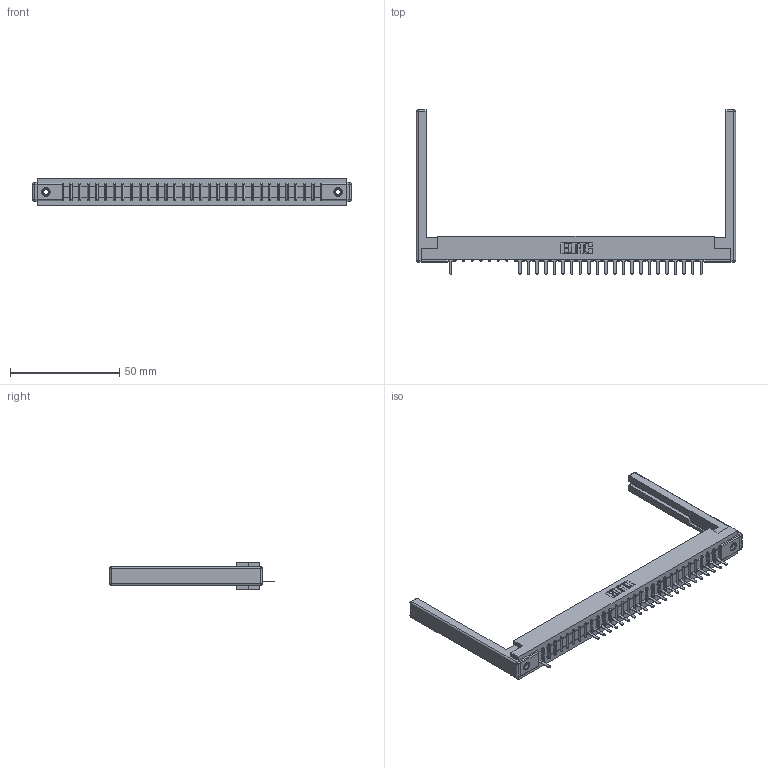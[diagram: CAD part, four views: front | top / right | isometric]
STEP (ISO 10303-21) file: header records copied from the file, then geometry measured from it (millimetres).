
FILE_DESCRIPTION (( 'STEP AP203' ), '1' );
FILE_NAME ('307-030-525-168.STEP', '2018-08-04T18:25:08', ( '' ), ( '' ), 'SwSTEP 2.0', 'SolidWorks 2016', '' );
FILE_SCHEMA (( 'CONFIG_CONTROL_DESIGN' ));
Length unit declared in the file: inch
Products named in the file (5): 307 Part_.156 Dia Mounting Holes; 307-290-001_525; 307-220-068; 345-250-001_345-250-001-102; 307-030-525-168
Assembly tree (28 placements, depth 2):
  307-030-525-168
    307 Part_.156 Dia Mounting Holes
    307-290-001_525  x23
    307-220-068  x2
    345-250-001_345-250-001-102  x2
Bounding box: 146.3 x 75.39 x 12.7 mm (x, y, z)
Volume: 19392.1 mm3; surface area: 19005.8 mm2
Topology: 28 solids, 28 shells, 1731 faces, 4887 edges, 3122 vertices
Faces by surface type: plane 1093, cylinder 552, sphere 70, cone 12, torus 4
Entity records: 29701 total; most frequent: CARTESIAN_POINT 4994, ORIENTED_EDGE 4976, DIRECTION 4874, EDGE_CURVE 2488, LINE 1902, VECTOR 1902, VERTEX_POINT 1606, AXIS2_PLACEMENT_3D 1486
